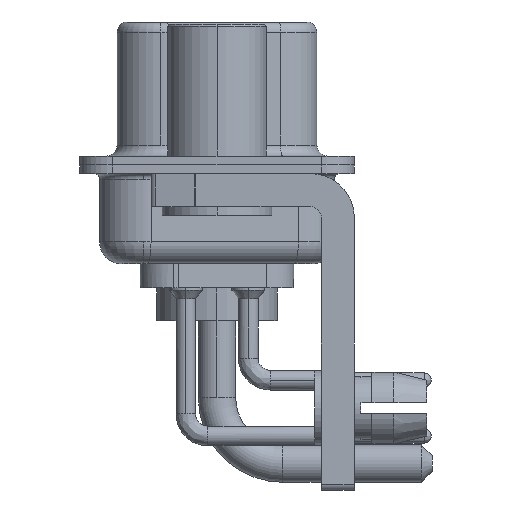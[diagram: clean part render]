
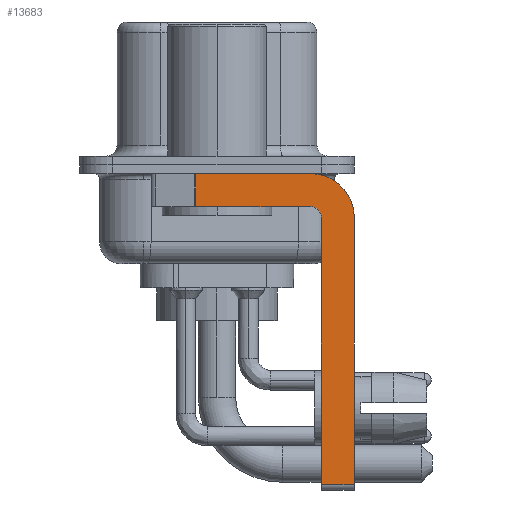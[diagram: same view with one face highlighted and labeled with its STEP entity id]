
A CAD part, left-side view. The second image highlights one B-rep face of the part: STEP entity #13683.
In plain terms, the highlighted planar face has unit normal (-1, 0, 0).
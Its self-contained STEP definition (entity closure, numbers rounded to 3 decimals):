
#44 = DIRECTION ( 'NONE',  ( 0., 0., 1. ) ) ;
#514 = AXIS2_PLACEMENT_3D ( 'NONE', #21373, #23741, #3367 ) ;
#755 = ORIENTED_EDGE ( 'NONE', *, *, #24095, .T. ) ;
#1614 = CARTESIAN_POINT ( 'NONE',  ( -2.9, -6.25, -14.55 ) ) ;
#1763 = ORIENTED_EDGE ( 'NONE', *, *, #11265, .F. ) ;
#2217 = DIRECTION ( 'NONE',  ( 0., 0., -1. ) ) ;
#2638 = DIRECTION ( 'NONE',  ( 0., -1., 0. ) ) ;
#2861 = EDGE_CURVE ( 'NONE', #25624, #28372, #25635, .T. ) ;
#3190 = EDGE_LOOP ( 'NONE', ( #8756, #19617, #22602, #21212, #18503, #755, #1763, #12843 ) ) ;
#3367 = DIRECTION ( 'NONE',  ( 0., 0., 1. ) ) ;
#3546 = CARTESIAN_POINT ( 'NONE',  ( -2.9, 0.978, -1.9 ) ) ;
#3730 = DIRECTION ( 'NONE',  ( 0., -1., 0. ) ) ;
#3861 = VECTOR ( 'NONE', #3730, 1000. ) ;
#4095 = CARTESIAN_POINT ( 'NONE',  ( -2.9, 0.978, -1.9 ) ) ;
#4924 = DIRECTION ( 'NONE',  ( 1., 0., 0. ) ) ;
#6023 = CARTESIAN_POINT ( 'NONE',  ( -2.9, -4.25, -1.9 ) ) ;
#6693 = PLANE ( 'NONE',  #9410 ) ;
#6827 = CARTESIAN_POINT ( 'NONE',  ( -2.9, -4.75, -14.55 ) ) ;
#6962 = LINE ( 'NONE', #20508, #18724 ) ;
#8031 = DIRECTION ( 'NONE',  ( 0., 0., -1. ) ) ;
#8756 = ORIENTED_EDGE ( 'NONE', *, *, #2861, .F. ) ;
#8894 = EDGE_CURVE ( 'NONE', #25624, #23308, #19185, .T. ) ;
#9110 = VERTEX_POINT ( 'NONE', #9316 ) ;
#9316 = CARTESIAN_POINT ( 'NONE',  ( -2.9, -4.75, -2.4 ) ) ;
#9410 = AXIS2_PLACEMENT_3D ( 'NONE', #11462, #4924, #2217 ) ;
#9826 = LINE ( 'NONE', #12202, #15493 ) ;
#10044 = DIRECTION ( 'NONE',  ( 0., 1., 0. ) ) ;
#10199 = CARTESIAN_POINT ( 'NONE',  ( -2.9, 0.978, -0.4 ) ) ;
#11265 = EDGE_CURVE ( 'NONE', #21631, #11437, #9826, .T. ) ;
#11437 = VERTEX_POINT ( 'NONE', #1614 ) ;
#11462 = CARTESIAN_POINT ( 'NONE',  ( -2.9, -4.25, -2.4 ) ) ;
#11946 = LINE ( 'NONE', #25496, #17672 ) ;
#12202 = CARTESIAN_POINT ( 'NONE',  ( -2.9, -6.25, -2.4 ) ) ;
#12787 = CARTESIAN_POINT ( 'NONE',  ( -2.9, -4.25, -2.4 ) ) ;
#12843 = ORIENTED_EDGE ( 'NONE', *, *, #19137, .F. ) ;
#13683 = ADVANCED_FACE ( 'NONE', ( #15914 ), #6693, .F. ) ;
#14437 = DIRECTION ( 'NONE',  ( 0., 0., -1. ) ) ;
#14575 = CARTESIAN_POINT ( 'NONE',  ( -2.9, -6.25, -2.4 ) ) ;
#14740 = DIRECTION ( 'NONE',  ( 0., 0., -1. ) ) ;
#14811 = LINE ( 'NONE', #6023, #29395 ) ;
#15493 = VECTOR ( 'NONE', #8031, 1000. ) ;
#15804 = VECTOR ( 'NONE', #14437, 1000. ) ;
#15914 = FACE_OUTER_BOUND ( 'NONE', #3190, .T. ) ;
#16014 = CARTESIAN_POINT ( 'NONE',  ( -2.9, -4.25, -0.4 ) ) ;
#16973 = EDGE_CURVE ( 'NONE', #19505, #23308, #14811, .T. ) ;
#17672 = VECTOR ( 'NONE', #44, 1000. ) ;
#18503 = ORIENTED_EDGE ( 'NONE', *, *, #22479, .F. ) ;
#18724 = VECTOR ( 'NONE', #2638, 1000. ) ;
#19137 = EDGE_CURVE ( 'NONE', #28372, #21631, #22801, .T. ) ;
#19185 = LINE ( 'NONE', #3546, #15804 ) ;
#19505 = VERTEX_POINT ( 'NONE', #20988 ) ;
#19617 = ORIENTED_EDGE ( 'NONE', *, *, #8894, .T. ) ;
#20317 = EDGE_CURVE ( 'NONE', #9110, #19505, #25715, .T. ) ;
#20508 = CARTESIAN_POINT ( 'NONE',  ( -2.9, -4.25, -14.55 ) ) ;
#20988 = CARTESIAN_POINT ( 'NONE',  ( -2.9, -4.25, -1.9 ) ) ;
#21212 = ORIENTED_EDGE ( 'NONE', *, *, #20317, .F. ) ;
#21373 = CARTESIAN_POINT ( 'NONE',  ( -2.9, -4.25, -2.4 ) ) ;
#21631 = VERTEX_POINT ( 'NONE', #14575 ) ;
#22479 = EDGE_CURVE ( 'NONE', #25418, #9110, #11946, .T. ) ;
#22602 = ORIENTED_EDGE ( 'NONE', *, *, #16973, .F. ) ;
#22801 = CIRCLE ( 'NONE', #23265, 2. ) ;
#23265 = AXIS2_PLACEMENT_3D ( 'NONE', #12787, #28130, #14740 ) ;
#23308 = VERTEX_POINT ( 'NONE', #4095 ) ;
#23741 = DIRECTION ( 'NONE',  ( -1., 0., 0. ) ) ;
#24095 = EDGE_CURVE ( 'NONE', #25418, #11437, #6962, .T. ) ;
#25418 = VERTEX_POINT ( 'NONE', #6827 ) ;
#25496 = CARTESIAN_POINT ( 'NONE',  ( -2.9, -4.75, -14.8 ) ) ;
#25624 = VERTEX_POINT ( 'NONE', #10199 ) ;
#25635 = LINE ( 'NONE', #28574, #3861 ) ;
#25715 = CIRCLE ( 'NONE', #514, 0.5 ) ;
#28130 = DIRECTION ( 'NONE',  ( 1., 0., 0. ) ) ;
#28372 = VERTEX_POINT ( 'NONE', #16014 ) ;
#28574 = CARTESIAN_POINT ( 'NONE',  ( -2.9, 3., -0.4 ) ) ;
#29395 = VECTOR ( 'NONE', #10044, 1000. ) ;
